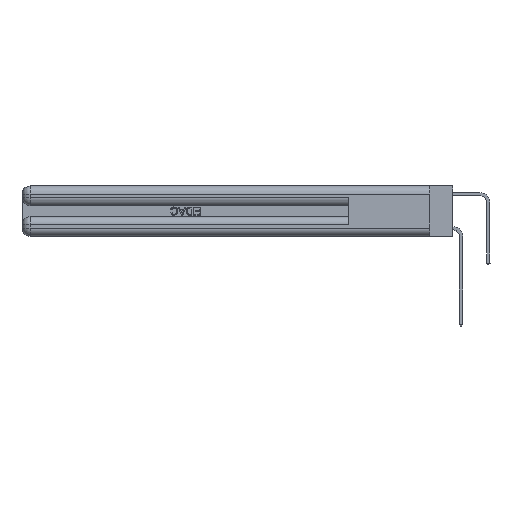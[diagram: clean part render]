
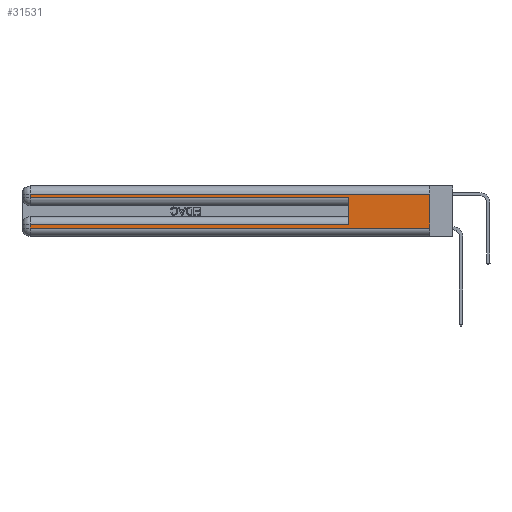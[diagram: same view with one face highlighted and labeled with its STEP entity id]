
A CAD part, left-side view. The second image highlights one B-rep face of the part: STEP entity #31531.
In plain terms, the highlighted planar face has unit normal (-1, 0, 0).
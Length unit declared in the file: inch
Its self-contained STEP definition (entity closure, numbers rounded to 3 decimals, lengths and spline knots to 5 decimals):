
#554 = ORIENTED_EDGE ( 'NONE', *, *, #30623, .T. ) ;
#659 = CARTESIAN_POINT ( 'NONE',  ( 0., 0., 0.06 ) ) ;
#801 = DIRECTION ( 'NONE',  ( 0., 0., -1. ) ) ;
#1598 = LINE ( 'NONE', #18429, #22374 ) ;
#1721 = VERTEX_POINT ( 'NONE', #32533 ) ;
#2176 = LINE ( 'NONE', #13098, #8330 ) ;
#3075 = CARTESIAN_POINT ( 'NONE',  ( 0., 0.6, 0.085 ) ) ;
#3949 = DIRECTION ( 'NONE',  ( 1., 0., 0. ) ) ;
#4944 = DIRECTION ( 'NONE',  ( 0., -1., 0. ) ) ;
#5145 = ORIENTED_EDGE ( 'NONE', *, *, #32843, .T. ) ;
#5148 = DIRECTION ( 'NONE',  ( 0., 1., 0. ) ) ;
#5624 = CARTESIAN_POINT ( 'NONE',  ( 0., 0., 0.06 ) ) ;
#6403 = CARTESIAN_POINT ( 'NONE',  ( 0., 0.6, 0.145 ) ) ;
#6805 = CARTESIAN_POINT ( 'NONE',  ( 0., 0.6, 0.285 ) ) ;
#6901 = ORIENTED_EDGE ( 'NONE', *, *, #20160, .T. ) ;
#8330 = VECTOR ( 'NONE', #4944, 39.37008 ) ;
#8754 = DIRECTION ( 'NONE',  ( 0., 0., -1. ) ) ;
#8989 = EDGE_LOOP ( 'NONE', ( #24032, #5145, #16164, #6901, #10149, #29365, #554, #12784 ) ) ;
#9442 = CARTESIAN_POINT ( 'NONE',  ( 0., 2.94, 0.37 ) ) ;
#9645 = VERTEX_POINT ( 'NONE', #35390 ) ;
#10149 = ORIENTED_EDGE ( 'NONE', *, *, #31043, .F. ) ;
#10436 = VERTEX_POINT ( 'NONE', #31371 ) ;
#11261 = VERTEX_POINT ( 'NONE', #5624 ) ;
#11771 = DIRECTION ( 'NONE',  ( 0., -1., 0. ) ) ;
#12226 = VERTEX_POINT ( 'NONE', #31338 ) ;
#12784 = ORIENTED_EDGE ( 'NONE', *, *, #25183, .T. ) ;
#13098 = CARTESIAN_POINT ( 'NONE',  ( 0., 0., 0.285 ) ) ;
#13654 = LINE ( 'NONE', #31002, #19277 ) ;
#13782 = VECTOR ( 'NONE', #8754, 39.37008 ) ;
#13960 = LINE ( 'NONE', #25947, #13782 ) ;
#14451 = VERTEX_POINT ( 'NONE', #3075 ) ;
#15840 = EDGE_CURVE ( 'NONE', #14451, #10436, #1598, .T. ) ;
#16039 = DIRECTION ( 'NONE',  ( 0., 1., 0. ) ) ;
#16164 = ORIENTED_EDGE ( 'NONE', *, *, #28797, .T. ) ;
#16511 = DIRECTION ( 'NONE',  ( 0., 0., -1. ) ) ;
#17677 = DIRECTION ( 'NONE',  ( 0., 0., 1. ) ) ;
#18221 = CARTESIAN_POINT ( 'NONE',  ( 0., 2.94, 0.06 ) ) ;
#18429 = CARTESIAN_POINT ( 'NONE',  ( 0., 0., 0.085 ) ) ;
#19277 = VECTOR ( 'NONE', #5148, 39.37008 ) ;
#19708 = LINE ( 'NONE', #659, #31541 ) ;
#20160 = EDGE_CURVE ( 'NONE', #9645, #28221, #2176, .T. ) ;
#20306 = VECTOR ( 'NONE', #20720, 39.37008 ) ;
#20720 = DIRECTION ( 'NONE',  ( 0., 0., -1. ) ) ;
#20809 = LINE ( 'NONE', #6403, #35719 ) ;
#21604 = VERTEX_POINT ( 'NONE', #18221 ) ;
#22374 = VECTOR ( 'NONE', #16039, 39.37008 ) ;
#23189 = FACE_OUTER_BOUND ( 'NONE', #8989, .T. ) ;
#23291 = VECTOR ( 'NONE', #16511, 39.37008 ) ;
#23501 = LINE ( 'NONE', #9442, #20306 ) ;
#23738 = CARTESIAN_POINT ( 'NONE',  ( 0., 0., 0.37 ) ) ;
#24032 = ORIENTED_EDGE ( 'NONE', *, *, #27289, .F. ) ;
#25121 = AXIS2_PLACEMENT_3D ( 'NONE', #23738, #3949, #801 ) ;
#25183 = EDGE_CURVE ( 'NONE', #21604, #11261, #19708, .T. ) ;
#25947 = CARTESIAN_POINT ( 'NONE',  ( 0., 0., 0.37 ) ) ;
#27289 = EDGE_CURVE ( 'NONE', #12226, #11261, #13960, .T. ) ;
#28221 = VERTEX_POINT ( 'NONE', #6805 ) ;
#28797 = EDGE_CURVE ( 'NONE', #1721, #9645, #35416, .T. ) ;
#29365 = ORIENTED_EDGE ( 'NONE', *, *, #15840, .T. ) ;
#29863 = CARTESIAN_POINT ( 'NONE',  ( 0., 2.94, 0.37 ) ) ;
#30623 = EDGE_CURVE ( 'NONE', #10436, #21604, #23501, .T. ) ;
#31002 = CARTESIAN_POINT ( 'NONE',  ( 0., 0., 0.31 ) ) ;
#31043 = EDGE_CURVE ( 'NONE', #14451, #28221, #20809, .T. ) ;
#31338 = CARTESIAN_POINT ( 'NONE',  ( 0., 0., 0.31 ) ) ;
#31371 = CARTESIAN_POINT ( 'NONE',  ( 0., 2.94, 0.085 ) ) ;
#31531 = ADVANCED_FACE ( 'NONE', ( #23189 ), #31844, .F. ) ;
#31541 = VECTOR ( 'NONE', #11771, 39.37008 ) ;
#31844 = PLANE ( 'NONE',  #25121 ) ;
#32533 = CARTESIAN_POINT ( 'NONE',  ( 0., 2.94, 0.31 ) ) ;
#32843 = EDGE_CURVE ( 'NONE', #12226, #1721, #13654, .T. ) ;
#35390 = CARTESIAN_POINT ( 'NONE',  ( 0., 2.94, 0.285 ) ) ;
#35416 = LINE ( 'NONE', #29863, #23291 ) ;
#35719 = VECTOR ( 'NONE', #17677, 39.37008 ) ;
